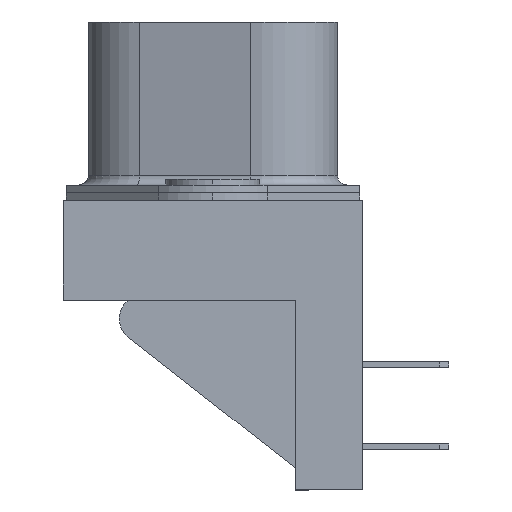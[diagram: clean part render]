
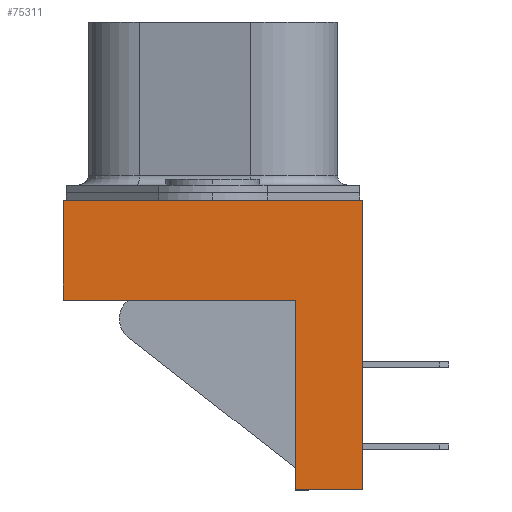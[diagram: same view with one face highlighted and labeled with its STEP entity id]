
A CAD part, left-side view. The second image highlights one B-rep face of the part: STEP entity #75311.
In plain terms, the highlighted planar face has unit normal (-1, 0, 0).
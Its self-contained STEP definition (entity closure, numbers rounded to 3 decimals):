
#663 = EDGE_CURVE ( 'NONE', #174545, #11351, #114804, .T. ) ;
#979 = LINE ( 'NONE', #15556, #150323 ) ;
#1517 = CARTESIAN_POINT ( 'NONE',  ( -4.125, -4.3, -5.2 ) ) ;
#11351 = VERTEX_POINT ( 'NONE', #13140 ) ;
#13140 = CARTESIAN_POINT ( 'NONE',  ( -4.125, 7.8, -5.2 ) ) ;
#14130 = EDGE_CURVE ( 'NONE', #41769, #174545, #82759, .T. ) ;
#14750 = DIRECTION ( 'NONE',  ( 0., 1., 0. ) ) ;
#15556 = CARTESIAN_POINT ( 'NONE',  ( -4.125, 7.8, -15.1 ) ) ;
#17349 = ORIENTED_EDGE ( 'NONE', *, *, #22342, .F. ) ;
#22342 = EDGE_CURVE ( 'NONE', #11351, #153628, #979, .T. ) ;
#22816 = CARTESIAN_POINT ( 'NONE',  ( -4.125, 7.8, -15.1 ) ) ;
#24794 = EDGE_CURVE ( 'NONE', #153628, #58839, #77476, .T. ) ;
#34698 = VECTOR ( 'NONE', #43537, 1000. ) ;
#34917 = VECTOR ( 'NONE', #50167, 1000. ) ;
#36464 = CARTESIAN_POINT ( 'NONE',  ( -4.125, 7.8, 0. ) ) ;
#41769 = VERTEX_POINT ( 'NONE', #74211 ) ;
#43537 = DIRECTION ( 'NONE',  ( 0., 0., 1. ) ) ;
#44964 = FACE_OUTER_BOUND ( 'NONE', #59554, .T. ) ;
#50167 = DIRECTION ( 'NONE',  ( 0., -1., 0. ) ) ;
#53251 = ORIENTED_EDGE ( 'NONE', *, *, #98294, .T. ) ;
#53477 = ORIENTED_EDGE ( 'NONE', *, *, #93988, .T. ) ;
#55071 = ORIENTED_EDGE ( 'NONE', *, *, #663, .F. ) ;
#56373 = CARTESIAN_POINT ( 'NONE',  ( -4.125, -7.8, 0. ) ) ;
#58839 = VERTEX_POINT ( 'NONE', #56373 ) ;
#59554 = EDGE_LOOP ( 'NONE', ( #55071, #129026, #53477, #53251, #86089, #17349 ) ) ;
#65971 = VECTOR ( 'NONE', #124308, 1000. ) ;
#71146 = CARTESIAN_POINT ( 'NONE',  ( -4.125, 7.8, -5.2 ) ) ;
#74211 = CARTESIAN_POINT ( 'NONE',  ( -4.125, -4.3, -15.1 ) ) ;
#75311 = ADVANCED_FACE ( 'NONE', ( #44964 ), #174708, .T. ) ;
#76280 = DIRECTION ( 'NONE',  ( 0., 0., 1. ) ) ;
#77476 = LINE ( 'NONE', #144797, #34917 ) ;
#78257 = VECTOR ( 'NONE', #14750, 1000. ) ;
#82759 = LINE ( 'NONE', #114536, #131113 ) ;
#85922 = DIRECTION ( 'NONE',  ( -1., 0., 0. ) ) ;
#86089 = ORIENTED_EDGE ( 'NONE', *, *, #24794, .F. ) ;
#93988 = EDGE_CURVE ( 'NONE', #41769, #138490, #178016, .T. ) ;
#98294 = EDGE_CURVE ( 'NONE', #138490, #58839, #123650, .T. ) ;
#114536 = CARTESIAN_POINT ( 'NONE',  ( -4.125, -4.3, -15.1 ) ) ;
#114804 = LINE ( 'NONE', #71146, #78257 ) ;
#123650 = LINE ( 'NONE', #179119, #34698 ) ;
#124308 = DIRECTION ( 'NONE',  ( 0., -1., 0. ) ) ;
#125632 = DIRECTION ( 'NONE',  ( 0., 0., 1. ) ) ;
#129026 = ORIENTED_EDGE ( 'NONE', *, *, #14130, .F. ) ;
#131113 = VECTOR ( 'NONE', #76280, 1000. ) ;
#138490 = VERTEX_POINT ( 'NONE', #163556 ) ;
#144797 = CARTESIAN_POINT ( 'NONE',  ( -4.125, 7.8, 0. ) ) ;
#150323 = VECTOR ( 'NONE', #125632, 1000. ) ;
#153628 = VERTEX_POINT ( 'NONE', #36464 ) ;
#157317 = AXIS2_PLACEMENT_3D ( 'NONE', #22816, #85922, #160182 ) ;
#160182 = DIRECTION ( 'NONE',  ( 0., -1., 0. ) ) ;
#163556 = CARTESIAN_POINT ( 'NONE',  ( -4.125, -7.8, -15.1 ) ) ;
#164349 = CARTESIAN_POINT ( 'NONE',  ( -4.125, 7.8, -15.1 ) ) ;
#174545 = VERTEX_POINT ( 'NONE', #1517 ) ;
#174708 = PLANE ( 'NONE',  #157317 ) ;
#178016 = LINE ( 'NONE', #164349, #65971 ) ;
#179119 = CARTESIAN_POINT ( 'NONE',  ( -4.125, -7.8, -15.1 ) ) ;
